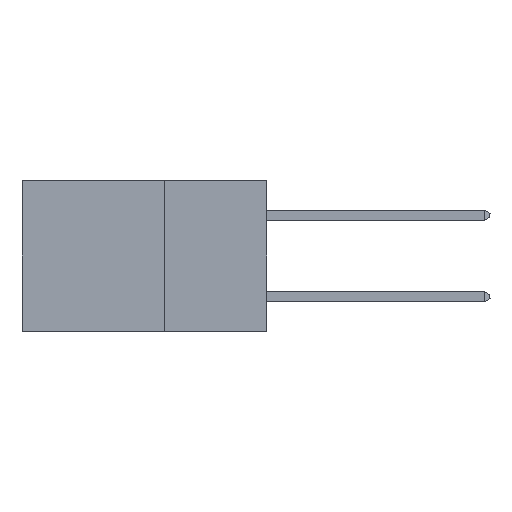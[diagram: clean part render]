
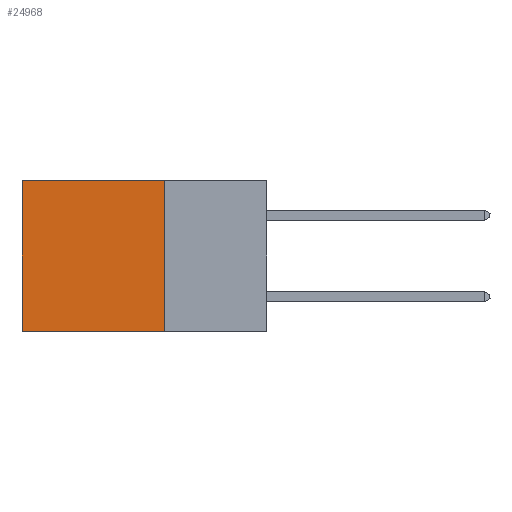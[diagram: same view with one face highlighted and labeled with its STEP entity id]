
A CAD part, left-side view. The second image highlights one B-rep face of the part: STEP entity #24968.
In plain terms, the highlighted planar face has unit normal (-1, 0, 0).
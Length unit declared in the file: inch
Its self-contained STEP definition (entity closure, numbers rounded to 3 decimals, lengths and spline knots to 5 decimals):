
#179 = DIRECTION ( 'NONE',  ( 0., 0., -1. ) ) ;
#451 = VECTOR ( 'NONE', #179, 39.37008 ) ;
#1057 = CARTESIAN_POINT ( 'NONE',  ( 0.2875, 0.25, 0. ) ) ;
#1210 = PLANE ( 'NONE',  #17958 ) ;
#1523 = VERTEX_POINT ( 'NONE', #19766 ) ;
#2908 = VERTEX_POINT ( 'NONE', #16973 ) ;
#2951 = DIRECTION ( 'NONE',  ( 1., 0., 0. ) ) ;
#3017 = CARTESIAN_POINT ( 'NONE',  ( 0.2875, 0.25, -0.37 ) ) ;
#3072 = CARTESIAN_POINT ( 'NONE',  ( 0.2875, 0.6, 0. ) ) ;
#4314 = VECTOR ( 'NONE', #11760, 39.37008 ) ;
#8415 = CARTESIAN_POINT ( 'NONE',  ( 0.2875, 0.25, -0.37 ) ) ;
#8557 = VECTOR ( 'NONE', #17613, 39.37008 ) ;
#8975 = ORIENTED_EDGE ( 'NONE', *, *, #15558, .T. ) ;
#11760 = DIRECTION ( 'NONE',  ( 0., 1., 0. ) ) ;
#11810 = VECTOR ( 'NONE', #17867, 39.37008 ) ;
#13733 = EDGE_CURVE ( 'NONE', #1523, #2908, #19357, .T. ) ;
#14785 = VERTEX_POINT ( 'NONE', #16675 ) ;
#14801 = LINE ( 'NONE', #3017, #8557 ) ;
#15558 = EDGE_CURVE ( 'NONE', #2908, #14785, #16713, .T. ) ;
#16189 = FACE_OUTER_BOUND ( 'NONE', #22713, .T. ) ;
#16675 = CARTESIAN_POINT ( 'NONE',  ( 0.2875, 0.6, -0.37 ) ) ;
#16713 = LINE ( 'NONE', #3072, #11810 ) ;
#16973 = CARTESIAN_POINT ( 'NONE',  ( 0.2875, 0.6, 0. ) ) ;
#17553 = DIRECTION ( 'NONE',  ( 0., 0., -1. ) ) ;
#17613 = DIRECTION ( 'NONE',  ( 0., 1., 0. ) ) ;
#17867 = DIRECTION ( 'NONE',  ( 0., 0., -1. ) ) ;
#17936 = CARTESIAN_POINT ( 'NONE',  ( 0.2875, 0.25, 0. ) ) ;
#17958 = AXIS2_PLACEMENT_3D ( 'NONE', #17936, #2951, #17553 ) ;
#18800 = LINE ( 'NONE', #21148, #451 ) ;
#19357 = LINE ( 'NONE', #1057, #4314 ) ;
#19766 = CARTESIAN_POINT ( 'NONE',  ( 0.2875, 0.25, 0. ) ) ;
#21139 = VERTEX_POINT ( 'NONE', #8415 ) ;
#21148 = CARTESIAN_POINT ( 'NONE',  ( 0.2875, 0.25, 0. ) ) ;
#21355 = ORIENTED_EDGE ( 'NONE', *, *, #25752, .F. ) ;
#22500 = ORIENTED_EDGE ( 'NONE', *, *, #13733, .T. ) ;
#22713 = EDGE_LOOP ( 'NONE', ( #8975, #21355, #24578, #22500 ) ) ;
#24578 = ORIENTED_EDGE ( 'NONE', *, *, #24674, .F. ) ;
#24674 = EDGE_CURVE ( 'NONE', #1523, #21139, #18800, .T. ) ;
#24968 = ADVANCED_FACE ( 'NONE', ( #16189 ), #1210, .F. ) ;
#25752 = EDGE_CURVE ( 'NONE', #21139, #14785, #14801, .T. ) ;
